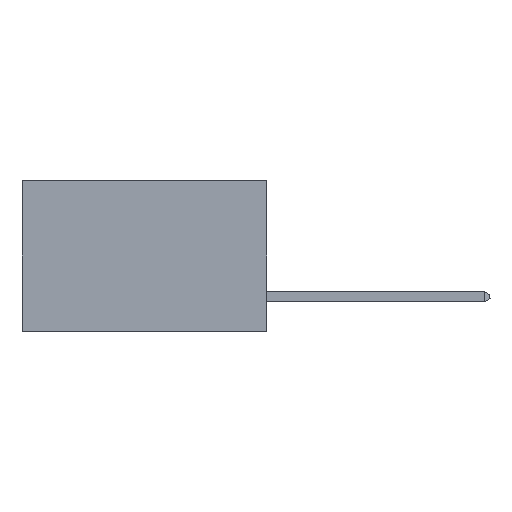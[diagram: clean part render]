
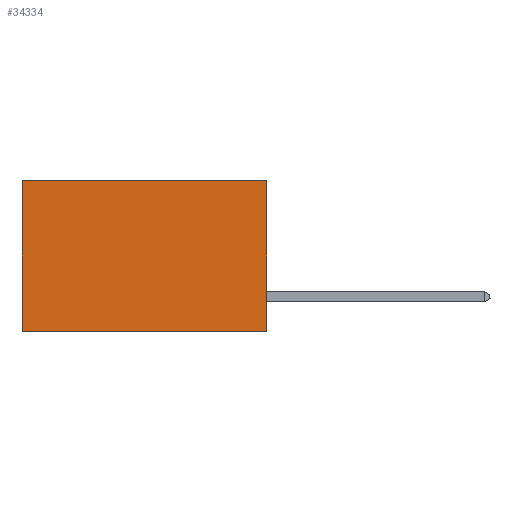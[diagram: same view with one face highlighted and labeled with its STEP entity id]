
A CAD part, left-side view. The second image highlights one B-rep face of the part: STEP entity #34334.
In plain terms, the highlighted planar face has unit normal (-1, 0, 0).
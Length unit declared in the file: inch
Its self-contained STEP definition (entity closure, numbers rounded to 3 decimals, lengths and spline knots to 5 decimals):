
#1557 = CARTESIAN_POINT ( 'NONE',  ( 0.2875, 0.6, -0.37 ) ) ;
#2214 = FACE_OUTER_BOUND ( 'NONE', #17648, .T. ) ;
#2569 = VECTOR ( 'NONE', #25272, 39.37008 ) ;
#4276 = DIRECTION ( 'NONE',  ( 0., 1., 0. ) ) ;
#4393 = VECTOR ( 'NONE', #25261, 39.37008 ) ;
#6582 = LINE ( 'NONE', #18326, #4393 ) ;
#7815 = ORIENTED_EDGE ( 'NONE', *, *, #33226, .T. ) ;
#8199 = CARTESIAN_POINT ( 'NONE',  ( 0.2875, 0., 0. ) ) ;
#10011 = ORIENTED_EDGE ( 'NONE', *, *, #22308, .T. ) ;
#11051 = CARTESIAN_POINT ( 'NONE',  ( 0.2875, 0., 0. ) ) ;
#11130 = DIRECTION ( 'NONE',  ( 1., 0., 0. ) ) ;
#11518 = LINE ( 'NONE', #20701, #18570 ) ;
#13443 = AXIS2_PLACEMENT_3D ( 'NONE', #8199, #11130, #30341 ) ;
#13801 = CARTESIAN_POINT ( 'NONE',  ( 0.2875, 0., -0.37 ) ) ;
#16097 = VECTOR ( 'NONE', #35456, 39.37008 ) ;
#17648 = EDGE_LOOP ( 'NONE', ( #10011, #22647, #25372, #7815 ) ) ;
#18086 = CARTESIAN_POINT ( 'NONE',  ( 0.2875, 0., 0. ) ) ;
#18326 = CARTESIAN_POINT ( 'NONE',  ( 0.2875, 0.6, 0. ) ) ;
#18570 = VECTOR ( 'NONE', #4276, 39.37008 ) ;
#19819 = EDGE_CURVE ( 'NONE', #33468, #30046, #35770, .T. ) ;
#20701 = CARTESIAN_POINT ( 'NONE',  ( 0.2875, 0., 0. ) ) ;
#22308 = EDGE_CURVE ( 'NONE', #35726, #31320, #6582, .T. ) ;
#22647 = ORIENTED_EDGE ( 'NONE', *, *, #34814, .F. ) ;
#25261 = DIRECTION ( 'NONE',  ( 0., 0., -1. ) ) ;
#25272 = DIRECTION ( 'NONE',  ( 0., 1., 0. ) ) ;
#25372 = ORIENTED_EDGE ( 'NONE', *, *, #19819, .F. ) ;
#25897 = CARTESIAN_POINT ( 'NONE',  ( 0.2875, 0.6, 0. ) ) ;
#29298 = LINE ( 'NONE', #13801, #2569 ) ;
#30046 = VERTEX_POINT ( 'NONE', #30354 ) ;
#30211 = PLANE ( 'NONE',  #13443 ) ;
#30341 = DIRECTION ( 'NONE',  ( 0., 0., -1. ) ) ;
#30354 = CARTESIAN_POINT ( 'NONE',  ( 0.2875, 0., -0.37 ) ) ;
#31320 = VERTEX_POINT ( 'NONE', #1557 ) ;
#33226 = EDGE_CURVE ( 'NONE', #33468, #35726, #11518, .T. ) ;
#33468 = VERTEX_POINT ( 'NONE', #11051 ) ;
#34334 = ADVANCED_FACE ( 'NONE', ( #2214 ), #30211, .F. ) ;
#34814 = EDGE_CURVE ( 'NONE', #30046, #31320, #29298, .T. ) ;
#35456 = DIRECTION ( 'NONE',  ( 0., 0., -1. ) ) ;
#35726 = VERTEX_POINT ( 'NONE', #25897 ) ;
#35770 = LINE ( 'NONE', #18086, #16097 ) ;
